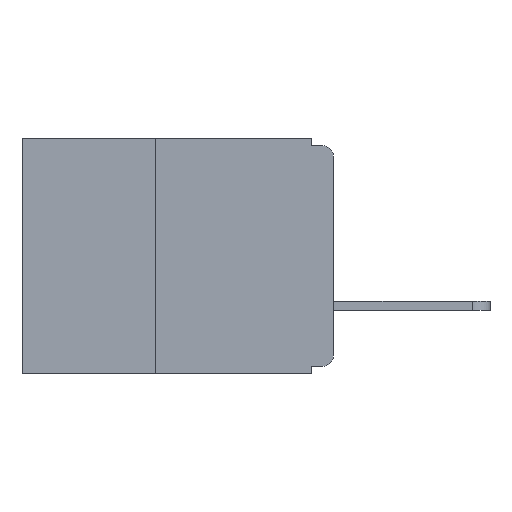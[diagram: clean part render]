
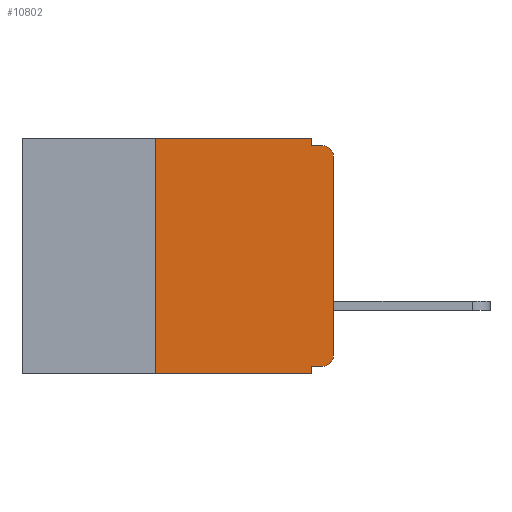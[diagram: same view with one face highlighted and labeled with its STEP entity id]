
A CAD part, left-side view. The second image highlights one B-rep face of the part: STEP entity #10802.
In plain terms, the highlighted planar face has unit normal (-1, 0, 0).
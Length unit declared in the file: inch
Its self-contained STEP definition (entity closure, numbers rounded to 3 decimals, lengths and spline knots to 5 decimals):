
#54 = ORIENTED_EDGE ( 'NONE', *, *, #2480, .F. ) ;
#111 = CARTESIAN_POINT ( 'NONE',  ( 0., 0.031, -0.33 ) ) ;
#245 = AXIS2_PLACEMENT_3D ( 'NONE', #9740, #11790, #9695 ) ;
#281 = VERTEX_POINT ( 'NONE', #12534 ) ;
#439 = LINE ( 'NONE', #8582, #2702 ) ;
#463 = VECTOR ( 'NONE', #7593, 39.37008 ) ;
#536 = VERTEX_POINT ( 'NONE', #8375 ) ;
#974 = DIRECTION ( 'NONE',  ( 0., 0., -1. ) ) ;
#1821 = DIRECTION ( 'NONE',  ( 0., 0., -1. ) ) ;
#2044 = CARTESIAN_POINT ( 'NONE',  ( 0., 0.031, -0.32 ) ) ;
#2163 = LINE ( 'NONE', #4954, #10051 ) ;
#2246 = VERTEX_POINT ( 'NONE', #6895 ) ;
#2480 = EDGE_CURVE ( 'NONE', #4391, #7550, #2163, .T. ) ;
#2556 = CARTESIAN_POINT ( 'NONE',  ( 0., 0.015, -0.32 ) ) ;
#2702 = VECTOR ( 'NONE', #9645, 39.37008 ) ;
#2777 = CARTESIAN_POINT ( 'NONE',  ( 0., 0.031, -0.01 ) ) ;
#2792 = DIRECTION ( 'NONE',  ( 0., 1., 0. ) ) ;
#2986 = ORIENTED_EDGE ( 'NONE', *, *, #6320, .T. ) ;
#3300 = DIRECTION ( 'NONE',  ( 0., 0., -1. ) ) ;
#4172 = CARTESIAN_POINT ( 'NONE',  ( 0., 0., 0. ) ) ;
#4239 = VERTEX_POINT ( 'NONE', #111 ) ;
#4391 = VERTEX_POINT ( 'NONE', #2556 ) ;
#4560 = ORIENTED_EDGE ( 'NONE', *, *, #6563, .T. ) ;
#4749 = ORIENTED_EDGE ( 'NONE', *, *, #5779, .F. ) ;
#4933 = LINE ( 'NONE', #13040, #12202 ) ;
#4954 = CARTESIAN_POINT ( 'NONE',  ( 0., 0., -0.32 ) ) ;
#5198 = ORIENTED_EDGE ( 'NONE', *, *, #8293, .T. ) ;
#5330 = CARTESIAN_POINT ( 'NONE',  ( 0., 0.25, -0.33 ) ) ;
#5413 = EDGE_LOOP ( 'NONE', ( #8883, #4560, #4749, #10778, #9224, #10950, #2986, #8819, #54, #5198 ) ) ;
#5529 = CIRCLE ( 'NONE', #245, 0.015 ) ;
#5569 = LINE ( 'NONE', #4172, #10758 ) ;
#5779 = EDGE_CURVE ( 'NONE', #6794, #10307, #11403, .T. ) ;
#6042 = CARTESIAN_POINT ( 'NONE',  ( 0., 0.031, 0. ) ) ;
#6135 = CARTESIAN_POINT ( 'NONE',  ( 0., 0.25, -0.33 ) ) ;
#6320 = EDGE_CURVE ( 'NONE', #7029, #4239, #439, .T. ) ;
#6347 = VECTOR ( 'NONE', #11729, 39.37008 ) ;
#6355 = DIRECTION ( 'NONE',  ( -1., 0., 0. ) ) ;
#6453 = EDGE_CURVE ( 'NONE', #281, #536, #5569, .T. ) ;
#6563 = EDGE_CURVE ( 'NONE', #536, #10307, #9286, .T. ) ;
#6597 = PLANE ( 'NONE',  #7064 ) ;
#6794 = VERTEX_POINT ( 'NONE', #2777 ) ;
#6895 = CARTESIAN_POINT ( 'NONE',  ( 0., 0.031, 0. ) ) ;
#7029 = VERTEX_POINT ( 'NONE', #6135 ) ;
#7064 = AXIS2_PLACEMENT_3D ( 'NONE', #10648, #11665, #8695 ) ;
#7175 = EDGE_CURVE ( 'NONE', #7029, #10109, #8444, .T. ) ;
#7315 = DIRECTION ( 'NONE',  ( 0., 0., 1. ) ) ;
#7550 = VERTEX_POINT ( 'NONE', #2044 ) ;
#7593 = DIRECTION ( 'NONE',  ( 0., -1., 0. ) ) ;
#8293 = EDGE_CURVE ( 'NONE', #4391, #281, #5529, .T. ) ;
#8375 = CARTESIAN_POINT ( 'NONE',  ( 0., 0., -0.025 ) ) ;
#8391 = CARTESIAN_POINT ( 'NONE',  ( 0., 0.015, -0.01 ) ) ;
#8444 = LINE ( 'NONE', #5330, #6347 ) ;
#8567 = FACE_OUTER_BOUND ( 'NONE', #5413, .T. ) ;
#8582 = CARTESIAN_POINT ( 'NONE',  ( 0., 0.437, -0.33 ) ) ;
#8608 = CARTESIAN_POINT ( 'NONE',  ( 0., 0.437, 0. ) ) ;
#8695 = DIRECTION ( 'NONE',  ( 0., 0., -1. ) ) ;
#8785 = VECTOR ( 'NONE', #974, 39.37008 ) ;
#8819 = ORIENTED_EDGE ( 'NONE', *, *, #12873, .F. ) ;
#8883 = ORIENTED_EDGE ( 'NONE', *, *, #6453, .T. ) ;
#8955 = EDGE_CURVE ( 'NONE', #2246, #6794, #10560, .T. ) ;
#9224 = ORIENTED_EDGE ( 'NONE', *, *, #10139, .F. ) ;
#9286 = CIRCLE ( 'NONE', #10771, 0.015 ) ;
#9571 = LINE ( 'NONE', #8608, #10872 ) ;
#9588 = CARTESIAN_POINT ( 'NONE',  ( 0., 0.015, -0.025 ) ) ;
#9645 = DIRECTION ( 'NONE',  ( 0., -1., 0. ) ) ;
#9695 = DIRECTION ( 'NONE',  ( 0., 0., -1. ) ) ;
#9740 = CARTESIAN_POINT ( 'NONE',  ( 0., 0.015, -0.305 ) ) ;
#10051 = VECTOR ( 'NONE', #2792, 39.37008 ) ;
#10109 = VERTEX_POINT ( 'NONE', #11718 ) ;
#10139 = EDGE_CURVE ( 'NONE', #10109, #2246, #9571, .T. ) ;
#10307 = VERTEX_POINT ( 'NONE', #8391 ) ;
#10560 = LINE ( 'NONE', #6042, #8785 ) ;
#10648 = CARTESIAN_POINT ( 'NONE',  ( 0., 0.437, 0. ) ) ;
#10758 = VECTOR ( 'NONE', #7315, 39.37008 ) ;
#10771 = AXIS2_PLACEMENT_3D ( 'NONE', #9588, #6355, #3300 ) ;
#10778 = ORIENTED_EDGE ( 'NONE', *, *, #8955, .F. ) ;
#10802 = ADVANCED_FACE ( 'NONE', ( #8567 ), #6597, .F. ) ;
#10872 = VECTOR ( 'NONE', #12520, 39.37008 ) ;
#10950 = ORIENTED_EDGE ( 'NONE', *, *, #7175, .F. ) ;
#11403 = LINE ( 'NONE', #13261, #463 ) ;
#11665 = DIRECTION ( 'NONE',  ( 1., 0., 0. ) ) ;
#11718 = CARTESIAN_POINT ( 'NONE',  ( 0., 0.25, 0. ) ) ;
#11729 = DIRECTION ( 'NONE',  ( 0., 0., 1. ) ) ;
#11790 = DIRECTION ( 'NONE',  ( -1., 0., 0. ) ) ;
#12202 = VECTOR ( 'NONE', #1821, 39.37008 ) ;
#12520 = DIRECTION ( 'NONE',  ( 0., -1., 0. ) ) ;
#12534 = CARTESIAN_POINT ( 'NONE',  ( 0., 0., -0.305 ) ) ;
#12873 = EDGE_CURVE ( 'NONE', #7550, #4239, #4933, .T. ) ;
#13040 = CARTESIAN_POINT ( 'NONE',  ( 0., 0.031, -0.33 ) ) ;
#13261 = CARTESIAN_POINT ( 'NONE',  ( 0., 0., -0.01 ) ) ;
